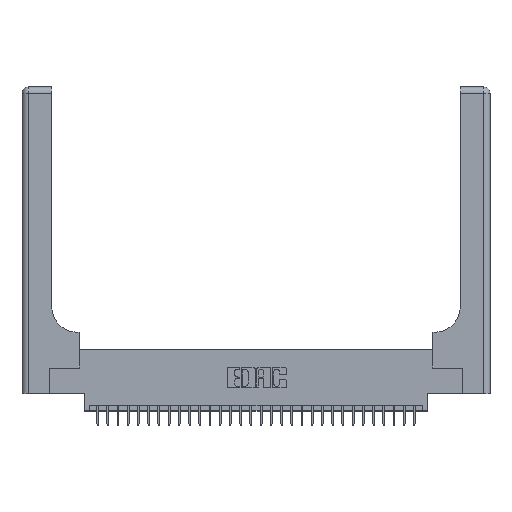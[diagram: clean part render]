
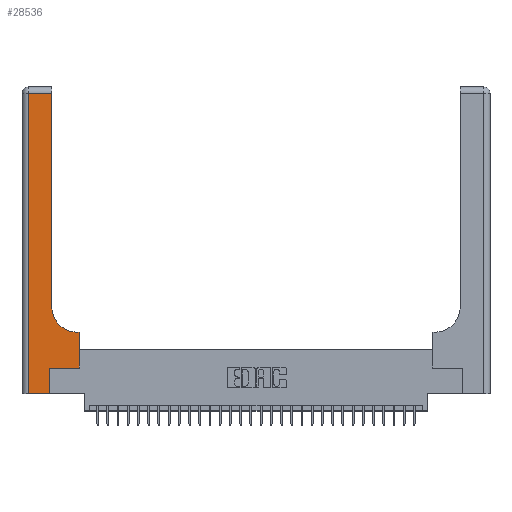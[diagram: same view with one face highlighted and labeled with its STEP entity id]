
A CAD part, top view. The second image highlights one B-rep face of the part: STEP entity #28536.
In plain terms, the highlighted planar face has unit normal (0, 0, 1).
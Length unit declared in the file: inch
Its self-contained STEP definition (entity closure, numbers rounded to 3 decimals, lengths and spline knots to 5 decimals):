
#683 = CARTESIAN_POINT ( 'NONE',  ( 0.2915, 0.85, 0.37 ) ) ;
#846 = CARTESIAN_POINT ( 'NONE',  ( 0.269, 0.25, 0.37 ) ) ;
#1266 = VECTOR ( 'NONE', #11097, 39.37008 ) ;
#1440 = VERTEX_POINT ( 'NONE', #683 ) ;
#1656 = DIRECTION ( 'NONE',  ( 0., 1., 0. ) ) ;
#2938 = CARTESIAN_POINT ( 'NONE',  ( 0.2915, 3., 0.37 ) ) ;
#3624 = PLANE ( 'NONE',  #18314 ) ;
#4126 = CARTESIAN_POINT ( 'NONE',  ( 0., 3., 0.37 ) ) ;
#4258 = ORIENTED_EDGE ( 'NONE', *, *, #7349, .T. ) ;
#4705 = VERTEX_POINT ( 'NONE', #24777 ) ;
#4880 = CIRCLE ( 'NONE', #7352, 0.25 ) ;
#5194 = LINE ( 'NONE', #2938, #13005 ) ;
#5591 = VECTOR ( 'NONE', #11196, 39.37008 ) ;
#6130 = LINE ( 'NONE', #25485, #1266 ) ;
#7301 = VECTOR ( 'NONE', #1656, 39.37008 ) ;
#7349 = EDGE_CURVE ( 'NONE', #30534, #4705, #14866, .T. ) ;
#7352 = AXIS2_PLACEMENT_3D ( 'NONE', #19715, #27356, #29644 ) ;
#7398 = CARTESIAN_POINT ( 'NONE',  ( 0.06, 3., 0.37 ) ) ;
#7423 = VECTOR ( 'NONE', #29784, 39.37008 ) ;
#7897 = LINE ( 'NONE', #846, #21684 ) ;
#8197 = ORIENTED_EDGE ( 'NONE', *, *, #31274, .T. ) ;
#8322 = EDGE_CURVE ( 'NONE', #24691, #24699, #6130, .T. ) ;
#9986 = DIRECTION ( 'NONE',  ( 0., -1., 0. ) ) ;
#10282 = LINE ( 'NONE', #24494, #30450 ) ;
#10480 = DIRECTION ( 'NONE',  ( 1., 0., 0. ) ) ;
#11097 = DIRECTION ( 'NONE',  ( -1., 0., 0. ) ) ;
#11196 = DIRECTION ( 'NONE',  ( -1., 0., 0. ) ) ;
#11913 = CARTESIAN_POINT ( 'NONE',  ( 0.2915, 2.94, 0.37 ) ) ;
#12725 = ORIENTED_EDGE ( 'NONE', *, *, #19620, .T. ) ;
#13005 = VECTOR ( 'NONE', #22563, 39.37008 ) ;
#13073 = EDGE_CURVE ( 'NONE', #4705, #13806, #15852, .T. ) ;
#13674 = LINE ( 'NONE', #28242, #7301 ) ;
#13806 = VERTEX_POINT ( 'NONE', #22618 ) ;
#14206 = VERTEX_POINT ( 'NONE', #19813 ) ;
#14866 = LINE ( 'NONE', #26866, #7423 ) ;
#15739 = ORIENTED_EDGE ( 'NONE', *, *, #24905, .T. ) ;
#15852 = LINE ( 'NONE', #23304, #5591 ) ;
#17846 = CARTESIAN_POINT ( 'NONE',  ( 0.5585, 0.25, 0.37 ) ) ;
#17938 = ORIENTED_EDGE ( 'NONE', *, *, #13073, .T. ) ;
#18116 = EDGE_CURVE ( 'NONE', #14206, #20206, #10282, .T. ) ;
#18314 = AXIS2_PLACEMENT_3D ( 'NONE', #4126, #20816, #30572 ) ;
#19462 = DIRECTION ( 'NONE',  ( 1., 0., 0. ) ) ;
#19620 = EDGE_CURVE ( 'NONE', #22075, #30534, #7897, .T. ) ;
#19715 = CARTESIAN_POINT ( 'NONE',  ( 0.5415, 0.85, 0.37 ) ) ;
#19759 = EDGE_CURVE ( 'NONE', #20206, #22075, #13674, .T. ) ;
#19813 = CARTESIAN_POINT ( 'NONE',  ( 0.06, 0., 0.37 ) ) ;
#20206 = VERTEX_POINT ( 'NONE', #21022 ) ;
#20387 = CARTESIAN_POINT ( 'NONE',  ( 0.269, 0.25, 0.37 ) ) ;
#20816 = DIRECTION ( 'NONE',  ( 0., 0., -1. ) ) ;
#21022 = CARTESIAN_POINT ( 'NONE',  ( 0.269, 0., 0.37 ) ) ;
#21684 = VECTOR ( 'NONE', #10480, 39.37008 ) ;
#22075 = VERTEX_POINT ( 'NONE', #20387 ) ;
#22563 = DIRECTION ( 'NONE',  ( 0., 1., 0. ) ) ;
#22618 = CARTESIAN_POINT ( 'NONE',  ( 0.5415, 0.6, 0.37 ) ) ;
#23049 = EDGE_LOOP ( 'NONE', ( #15739, #23851, #8197, #23889, #25136, #12725, #4258, #17938, #31264 ) ) ;
#23304 = CARTESIAN_POINT ( 'NONE',  ( 0.2915, 0.6, 0.37 ) ) ;
#23537 = VECTOR ( 'NONE', #9986, 39.37008 ) ;
#23851 = ORIENTED_EDGE ( 'NONE', *, *, #8322, .T. ) ;
#23889 = ORIENTED_EDGE ( 'NONE', *, *, #18116, .T. ) ;
#24494 = CARTESIAN_POINT ( 'NONE',  ( 0., 0., 0.37 ) ) ;
#24532 = EDGE_CURVE ( 'NONE', #13806, #1440, #4880, .T. ) ;
#24691 = VERTEX_POINT ( 'NONE', #11913 ) ;
#24699 = VERTEX_POINT ( 'NONE', #26647 ) ;
#24777 = CARTESIAN_POINT ( 'NONE',  ( 0.5585, 0.6, 0.37 ) ) ;
#24905 = EDGE_CURVE ( 'NONE', #1440, #24691, #5194, .T. ) ;
#25136 = ORIENTED_EDGE ( 'NONE', *, *, #19759, .T. ) ;
#25485 = CARTESIAN_POINT ( 'NONE',  ( 0., 2.94, 0.37 ) ) ;
#26647 = CARTESIAN_POINT ( 'NONE',  ( 0.06, 2.94, 0.37 ) ) ;
#26866 = CARTESIAN_POINT ( 'NONE',  ( 0.5585, 0.25, 0.37 ) ) ;
#27356 = DIRECTION ( 'NONE',  ( 0., 0., -1. ) ) ;
#28242 = CARTESIAN_POINT ( 'NONE',  ( 0.269, 0., 0.37 ) ) ;
#28536 = ADVANCED_FACE ( 'NONE', ( #30898 ), #3624, .F. ) ;
#29542 = LINE ( 'NONE', #7398, #23537 ) ;
#29644 = DIRECTION ( 'NONE',  ( 1., 0., 0. ) ) ;
#29784 = DIRECTION ( 'NONE',  ( 0., 1., 0. ) ) ;
#30450 = VECTOR ( 'NONE', #19462, 39.37008 ) ;
#30534 = VERTEX_POINT ( 'NONE', #17846 ) ;
#30572 = DIRECTION ( 'NONE',  ( -1., 0., 0. ) ) ;
#30898 = FACE_OUTER_BOUND ( 'NONE', #23049, .T. ) ;
#31264 = ORIENTED_EDGE ( 'NONE', *, *, #24532, .T. ) ;
#31274 = EDGE_CURVE ( 'NONE', #24699, #14206, #29542, .T. ) ;
